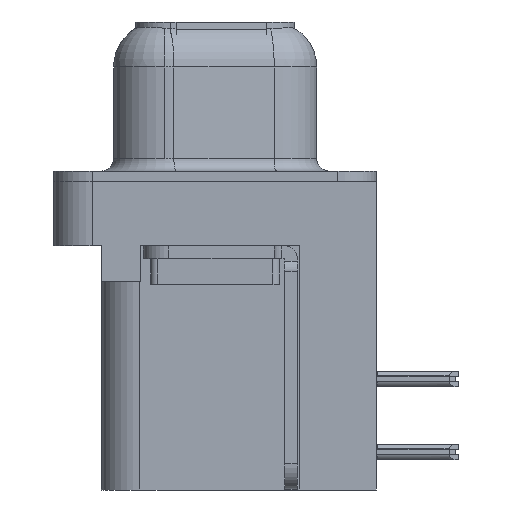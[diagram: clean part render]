
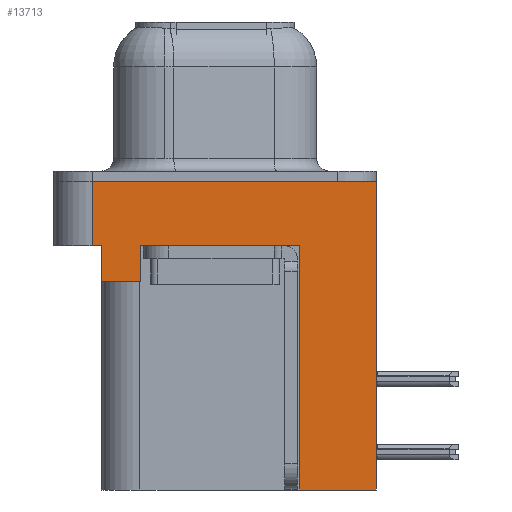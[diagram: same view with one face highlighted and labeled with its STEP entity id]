
A CAD part, left-side view. The second image highlights one B-rep face of the part: STEP entity #13713.
In plain terms, the highlighted planar face has unit normal (-1, 0, 0).
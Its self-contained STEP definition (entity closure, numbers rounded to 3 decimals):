
#627 = CARTESIAN_POINT ( 'NONE',  ( -2.91, 4.425, -2.5 ) ) ;
#692 = ORIENTED_EDGE ( 'NONE', *, *, #6129, .T. ) ;
#812 = VECTOR ( 'NONE', #26565, 1000. ) ;
#855 = DIRECTION ( 'NONE',  ( 0., 0., 1. ) ) ;
#1459 = DIRECTION ( 'NONE',  ( 0., 0., 1. ) ) ;
#1655 = DIRECTION ( 'NONE',  ( 0., 0., 1. ) ) ;
#1720 = ORIENTED_EDGE ( 'NONE', *, *, #5974, .F. ) ;
#2617 = VECTOR ( 'NONE', #855, 1000. ) ;
#2993 = ORIENTED_EDGE ( 'NONE', *, *, #19420, .F. ) ;
#3701 = CARTESIAN_POINT ( 'NONE',  ( -2.91, 4.775, 0. ) ) ;
#4775 = EDGE_CURVE ( 'NONE', #24720, #28339, #25884, .T. ) ;
#5595 = EDGE_CURVE ( 'NONE', #26640, #35073, #14406, .T. ) ;
#5816 = CARTESIAN_POINT ( 'NONE',  ( -2.91, -6.275, -12. ) ) ;
#5974 = EDGE_CURVE ( 'NONE', #19213, #33077, #20086, .T. ) ;
#6129 = EDGE_CURVE ( 'NONE', #31153, #24720, #34487, .T. ) ;
#6262 = LINE ( 'NONE', #35697, #15550 ) ;
#7190 = DIRECTION ( 'NONE',  ( -1., 0., 0. ) ) ;
#8830 = AXIS2_PLACEMENT_3D ( 'NONE', #18828, #7190, #1459 ) ;
#8849 = CARTESIAN_POINT ( 'NONE',  ( -2.91, 4.425, -3.9 ) ) ;
#9434 = EDGE_CURVE ( 'NONE', #26640, #20639, #33184, .T. ) ;
#9622 = EDGE_LOOP ( 'NONE', ( #12613, #29424, #33642, #2993, #12749, #692, #30570, #29336, #1720, #30874 ) ) ;
#10054 = VECTOR ( 'NONE', #31502, 1000. ) ;
#10349 = PLANE ( 'NONE',  #8830 ) ;
#10413 = DIRECTION ( 'NONE',  ( 0., 0., 1. ) ) ;
#11148 = EDGE_CURVE ( 'NONE', #19213, #32014, #18468, .T. ) ;
#11728 = VECTOR ( 'NONE', #12441, 1000. ) ;
#12441 = DIRECTION ( 'NONE',  ( 0., 1., 0. ) ) ;
#12613 = ORIENTED_EDGE ( 'NONE', *, *, #34133, .F. ) ;
#12749 = ORIENTED_EDGE ( 'NONE', *, *, #31331, .F. ) ;
#12858 = DIRECTION ( 'NONE',  ( 0., 0., 1. ) ) ;
#13156 = CARTESIAN_POINT ( 'NONE',  ( -2.91, -3.295, -2.5 ) ) ;
#13713 = ADVANCED_FACE ( 'NONE', ( #34147 ), #10349, .T. ) ;
#14037 = LINE ( 'NONE', #26823, #30637 ) ;
#14406 = LINE ( 'NONE', #20981, #35398 ) ;
#15275 = VECTOR ( 'NONE', #34926, 1000. ) ;
#15550 = VECTOR ( 'NONE', #28389, 1000. ) ;
#17465 = VECTOR ( 'NONE', #10413, 1000. ) ;
#18080 = CARTESIAN_POINT ( 'NONE',  ( -2.91, -6.275, 0. ) ) ;
#18096 = EDGE_CURVE ( 'NONE', #33077, #28339, #6262, .T. ) ;
#18468 = LINE ( 'NONE', #20712, #2617 ) ;
#18828 = CARTESIAN_POINT ( 'NONE',  ( -2.91, -6.275, -2.5 ) ) ;
#19213 = VERTEX_POINT ( 'NONE', #5816 ) ;
#19420 = EDGE_CURVE ( 'NONE', #30134, #20639, #14037, .T. ) ;
#20086 = LINE ( 'NONE', #34714, #11728 ) ;
#20639 = VERTEX_POINT ( 'NONE', #627 ) ;
#20712 = CARTESIAN_POINT ( 'NONE',  ( -2.91, -6.275, -2.5 ) ) ;
#20976 = VECTOR ( 'NONE', #33465, 1000. ) ;
#20981 = CARTESIAN_POINT ( 'NONE',  ( -2.91, 4.775, -2.5 ) ) ;
#21448 = CARTESIAN_POINT ( 'NONE',  ( -2.91, 4.775, -2.5 ) ) ;
#23055 = CARTESIAN_POINT ( 'NONE',  ( -2.91, -6.275, 0. ) ) ;
#24720 = VERTEX_POINT ( 'NONE', #35665 ) ;
#24840 = CARTESIAN_POINT ( 'NONE',  ( -2.91, 4.425, -3.9 ) ) ;
#24973 = LINE ( 'NONE', #8849, #10054 ) ;
#25307 = LINE ( 'NONE', #18080, #15275 ) ;
#25884 = LINE ( 'NONE', #26804, #812 ) ;
#26565 = DIRECTION ( 'NONE',  ( 0., -1., 0. ) ) ;
#26640 = VERTEX_POINT ( 'NONE', #21448 ) ;
#26804 = CARTESIAN_POINT ( 'NONE',  ( -2.91, -6.275, -2.5 ) ) ;
#26823 = CARTESIAN_POINT ( 'NONE',  ( -2.91, 4.425, -3.9 ) ) ;
#28339 = VERTEX_POINT ( 'NONE', #13156 ) ;
#28389 = DIRECTION ( 'NONE',  ( 0., 0., 1. ) ) ;
#29336 = ORIENTED_EDGE ( 'NONE', *, *, #18096, .F. ) ;
#29424 = ORIENTED_EDGE ( 'NONE', *, *, #5595, .F. ) ;
#30134 = VERTEX_POINT ( 'NONE', #24840 ) ;
#30516 = CARTESIAN_POINT ( 'NONE',  ( -2.91, -6.275, -2.5 ) ) ;
#30570 = ORIENTED_EDGE ( 'NONE', *, *, #4775, .T. ) ;
#30637 = VECTOR ( 'NONE', #1655, 1000. ) ;
#30874 = ORIENTED_EDGE ( 'NONE', *, *, #11148, .T. ) ;
#31017 = CARTESIAN_POINT ( 'NONE',  ( -2.91, 2.895, -3.9 ) ) ;
#31153 = VERTEX_POINT ( 'NONE', #31017 ) ;
#31331 = EDGE_CURVE ( 'NONE', #31153, #30134, #24973, .T. ) ;
#31502 = DIRECTION ( 'NONE',  ( 0., 1., 0. ) ) ;
#32014 = VERTEX_POINT ( 'NONE', #23055 ) ;
#32969 = CARTESIAN_POINT ( 'NONE',  ( -2.91, -3.295, -12. ) ) ;
#33077 = VERTEX_POINT ( 'NONE', #32969 ) ;
#33184 = LINE ( 'NONE', #30516, #20976 ) ;
#33465 = DIRECTION ( 'NONE',  ( 0., -1., 0. ) ) ;
#33642 = ORIENTED_EDGE ( 'NONE', *, *, #9434, .T. ) ;
#34133 = EDGE_CURVE ( 'NONE', #35073, #32014, #25307, .T. ) ;
#34147 = FACE_OUTER_BOUND ( 'NONE', #9622, .T. ) ;
#34487 = LINE ( 'NONE', #35255, #17465 ) ;
#34714 = CARTESIAN_POINT ( 'NONE',  ( -2.91, -3.295, -12. ) ) ;
#34926 = DIRECTION ( 'NONE',  ( 0., -1., 0. ) ) ;
#35073 = VERTEX_POINT ( 'NONE', #3701 ) ;
#35255 = CARTESIAN_POINT ( 'NONE',  ( -2.91, 2.895, -3.9 ) ) ;
#35398 = VECTOR ( 'NONE', #12858, 1000. ) ;
#35665 = CARTESIAN_POINT ( 'NONE',  ( -2.91, 2.895, -2.5 ) ) ;
#35697 = CARTESIAN_POINT ( 'NONE',  ( -2.91, -3.295, -12. ) ) ;
